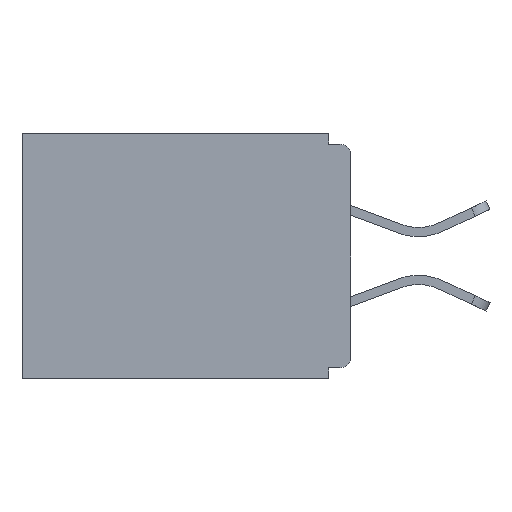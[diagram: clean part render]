
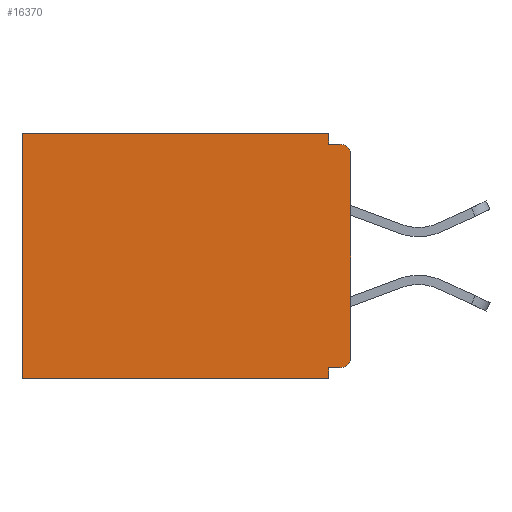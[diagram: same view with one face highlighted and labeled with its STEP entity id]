
A CAD part, left-side view. The second image highlights one B-rep face of the part: STEP entity #16370.
In plain terms, the highlighted planar face has unit normal (-1, 0, 0).
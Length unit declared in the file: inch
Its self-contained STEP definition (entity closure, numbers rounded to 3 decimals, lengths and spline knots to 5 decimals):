
#33 = VECTOR ( 'NONE', #11186, 39.37008 ) ;
#458 = AXIS2_PLACEMENT_3D ( 'NONE', #18896, #8520, #3585 ) ;
#495 = LINE ( 'NONE', #13297, #16914 ) ;
#682 = DIRECTION ( 'NONE',  ( -1., 0., 0. ) ) ;
#737 = VECTOR ( 'NONE', #20275, 39.37008 ) ;
#875 = EDGE_CURVE ( 'NONE', #19583, #15327, #4940, .T. ) ;
#1128 = ORIENTED_EDGE ( 'NONE', *, *, #4272, .T. ) ;
#1416 = CARTESIAN_POINT ( 'NONE',  ( 0.298, 0.031, -0.343 ) ) ;
#1509 = DIRECTION ( 'NONE',  ( 0., 0., -1. ) ) ;
#1970 = EDGE_CURVE ( 'NONE', #5703, #17993, #5464, .T. ) ;
#2157 = EDGE_CURVE ( 'NONE', #9030, #16214, #2640, .T. ) ;
#2640 = LINE ( 'NONE', #13058, #5059 ) ;
#3147 = DIRECTION ( 'NONE',  ( 0., 1., 0. ) ) ;
#3167 = DIRECTION ( 'NONE',  ( 1., 0., 0. ) ) ;
#3585 = DIRECTION ( 'NONE',  ( 0., 0., -1. ) ) ;
#3710 = DIRECTION ( 'NONE',  ( 0., 0., -1. ) ) ;
#4221 = DIRECTION ( 'NONE',  ( 0., 0., -1. ) ) ;
#4272 = EDGE_CURVE ( 'NONE', #5703, #16214, #11530, .T. ) ;
#4418 = ORIENTED_EDGE ( 'NONE', *, *, #12033, .F. ) ;
#4526 = EDGE_CURVE ( 'NONE', #12326, #16957, #495, .T. ) ;
#4595 = CARTESIAN_POINT ( 'NONE',  ( 0.298, 0., -0.03 ) ) ;
#4601 = LINE ( 'NONE', #13311, #33 ) ;
#4644 = VECTOR ( 'NONE', #13538, 39.37008 ) ;
#4940 = LINE ( 'NONE', #20392, #4644 ) ;
#5059 = VECTOR ( 'NONE', #6271, 39.37008 ) ;
#5168 = EDGE_CURVE ( 'NONE', #9030, #20563, #16895, .T. ) ;
#5464 = LINE ( 'NONE', #19852, #21642 ) ;
#5703 = VERTEX_POINT ( 'NONE', #15194 ) ;
#6271 = DIRECTION ( 'NONE',  ( 0., 0., -1. ) ) ;
#6319 = EDGE_LOOP ( 'NONE', ( #10648, #10353, #4418, #16750, #22041, #20399, #8764, #19201, #1128, #16605 ) ) ;
#6447 = CARTESIAN_POINT ( 'NONE',  ( 0.298, 0.031, -0.328 ) ) ;
#7611 = VECTOR ( 'NONE', #3710, 39.37008 ) ;
#7622 = VERTEX_POINT ( 'NONE', #10622 ) ;
#8520 = DIRECTION ( 'NONE',  ( -1., 0., 0. ) ) ;
#8764 = ORIENTED_EDGE ( 'NONE', *, *, #14777, .F. ) ;
#9030 = VERTEX_POINT ( 'NONE', #4595 ) ;
#9185 = CARTESIAN_POINT ( 'NONE',  ( 0.298, 0.015, -0.313 ) ) ;
#10353 = ORIENTED_EDGE ( 'NONE', *, *, #22342, .F. ) ;
#10622 = CARTESIAN_POINT ( 'NONE',  ( 0.298, 0.031, -0.015 ) ) ;
#10648 = ORIENTED_EDGE ( 'NONE', *, *, #5168, .T. ) ;
#11068 = FACE_OUTER_BOUND ( 'NONE', #6319, .T. ) ;
#11164 = CARTESIAN_POINT ( 'NONE',  ( 0.298, 0.46, -0.343 ) ) ;
#11186 = DIRECTION ( 'NONE',  ( 0., 0., -1. ) ) ;
#11530 = CIRCLE ( 'NONE', #20422, 0.015 ) ;
#11556 = CARTESIAN_POINT ( 'NONE',  ( 0.298, 0.46, 0. ) ) ;
#12013 = DIRECTION ( 'NONE',  ( 0., -1., 0. ) ) ;
#12033 = EDGE_CURVE ( 'NONE', #19583, #7622, #20330, .T. ) ;
#12326 = VERTEX_POINT ( 'NONE', #1416 ) ;
#12734 = AXIS2_PLACEMENT_3D ( 'NONE', #13461, #3167, #1509 ) ;
#13058 = CARTESIAN_POINT ( 'NONE',  ( 0.298, 0., 0. ) ) ;
#13297 = CARTESIAN_POINT ( 'NONE',  ( 0.298, 0., -0.343 ) ) ;
#13311 = CARTESIAN_POINT ( 'NONE',  ( 0.298, 0.46, 0. ) ) ;
#13461 = CARTESIAN_POINT ( 'NONE',  ( 0.298, 0., 0. ) ) ;
#13538 = DIRECTION ( 'NONE',  ( 0., 1., 0. ) ) ;
#14004 = CARTESIAN_POINT ( 'NONE',  ( 0.298, 0.031, -0.343 ) ) ;
#14238 = CARTESIAN_POINT ( 'NONE',  ( 0.298, 0.031, 0. ) ) ;
#14383 = CARTESIAN_POINT ( 'NONE',  ( 0.298, 0.015, -0.015 ) ) ;
#14777 = EDGE_CURVE ( 'NONE', #17993, #12326, #19668, .T. ) ;
#14817 = CARTESIAN_POINT ( 'NONE',  ( 0.298, 0., -0.313 ) ) ;
#15044 = DIRECTION ( 'NONE',  ( 0., 1., 0. ) ) ;
#15194 = CARTESIAN_POINT ( 'NONE',  ( 0.298, 0.015, -0.328 ) ) ;
#15327 = VERTEX_POINT ( 'NONE', #11556 ) ;
#15414 = CARTESIAN_POINT ( 'NONE',  ( 0.298, 0.031, -0.343 ) ) ;
#16214 = VERTEX_POINT ( 'NONE', #14817 ) ;
#16370 = ADVANCED_FACE ( 'NONE', ( #11068 ), #20558, .F. ) ;
#16605 = ORIENTED_EDGE ( 'NONE', *, *, #2157, .F. ) ;
#16750 = ORIENTED_EDGE ( 'NONE', *, *, #875, .T. ) ;
#16895 = CIRCLE ( 'NONE', #458, 0.015 ) ;
#16914 = VECTOR ( 'NONE', #15044, 39.37008 ) ;
#16957 = VERTEX_POINT ( 'NONE', #11164 ) ;
#17993 = VERTEX_POINT ( 'NONE', #6447 ) ;
#18665 = LINE ( 'NONE', #20833, #19774 ) ;
#18896 = CARTESIAN_POINT ( 'NONE',  ( 0.298, 0.015, -0.03 ) ) ;
#19201 = ORIENTED_EDGE ( 'NONE', *, *, #1970, .F. ) ;
#19583 = VERTEX_POINT ( 'NONE', #14238 ) ;
#19668 = LINE ( 'NONE', #15414, #737 ) ;
#19774 = VECTOR ( 'NONE', #12013, 39.37008 ) ;
#19852 = CARTESIAN_POINT ( 'NONE',  ( 0.298, 0., -0.328 ) ) ;
#20275 = DIRECTION ( 'NONE',  ( 0., 0., -1. ) ) ;
#20330 = LINE ( 'NONE', #14004, #7611 ) ;
#20392 = CARTESIAN_POINT ( 'NONE',  ( 0.298, 0., 0. ) ) ;
#20399 = ORIENTED_EDGE ( 'NONE', *, *, #4526, .F. ) ;
#20422 = AXIS2_PLACEMENT_3D ( 'NONE', #9185, #682, #4221 ) ;
#20558 = PLANE ( 'NONE',  #12734 ) ;
#20563 = VERTEX_POINT ( 'NONE', #14383 ) ;
#20833 = CARTESIAN_POINT ( 'NONE',  ( 0.298, 0., -0.015 ) ) ;
#21642 = VECTOR ( 'NONE', #3147, 39.37008 ) ;
#22041 = ORIENTED_EDGE ( 'NONE', *, *, #22148, .T. ) ;
#22148 = EDGE_CURVE ( 'NONE', #15327, #16957, #4601, .T. ) ;
#22342 = EDGE_CURVE ( 'NONE', #7622, #20563, #18665, .T. ) ;
